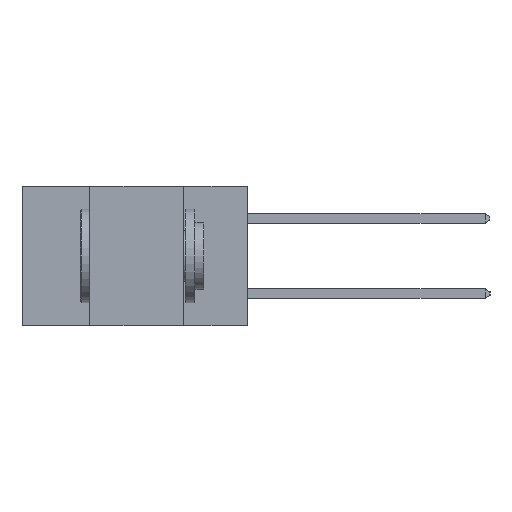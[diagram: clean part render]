
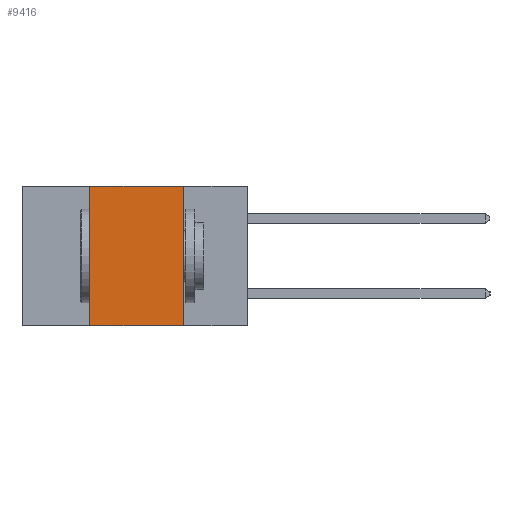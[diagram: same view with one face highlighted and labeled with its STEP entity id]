
A CAD part, left-side view. The second image highlights one B-rep face of the part: STEP entity #9416.
In plain terms, the highlighted planar face has unit normal (-1, 0, 0).
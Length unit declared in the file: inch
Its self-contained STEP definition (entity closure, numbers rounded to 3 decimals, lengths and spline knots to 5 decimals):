
#173 = VERTEX_POINT ( 'NONE', #4301 ) ;
#774 = LINE ( 'NONE', #1029, #2455 ) ;
#1029 = CARTESIAN_POINT ( 'NONE',  ( 0., 0.17, -0.37 ) ) ;
#1184 = CARTESIAN_POINT ( 'NONE',  ( 0., 0.17, 0. ) ) ;
#1533 = PLANE ( 'NONE',  #6991 ) ;
#1644 = LINE ( 'NONE', #10859, #11540 ) ;
#2072 = FACE_OUTER_BOUND ( 'NONE', #11758, .T. ) ;
#2455 = VECTOR ( 'NONE', #7136, 39.37008 ) ;
#2493 = CARTESIAN_POINT ( 'NONE',  ( 0., 0.6, 0. ) ) ;
#2840 = EDGE_CURVE ( 'NONE', #9882, #2846, #774, .T. ) ;
#2846 = VERTEX_POINT ( 'NONE', #10023 ) ;
#2974 = CARTESIAN_POINT ( 'NONE',  ( 0., 0.6, -0.37 ) ) ;
#3141 = LINE ( 'NONE', #6116, #10798 ) ;
#3213 = ORIENTED_EDGE ( 'NONE', *, *, #2840, .F. ) ;
#4301 = CARTESIAN_POINT ( 'NONE',  ( 0., 0.42, -0.37 ) ) ;
#4925 = LINE ( 'NONE', #2974, #12221 ) ;
#5420 = DIRECTION ( 'NONE',  ( 0., 0., -1. ) ) ;
#6071 = EDGE_CURVE ( 'NONE', #173, #8534, #1644, .T. ) ;
#6075 = DIRECTION ( 'NONE',  ( 0., -1., 0. ) ) ;
#6116 = CARTESIAN_POINT ( 'NONE',  ( 0., 0.6, 0. ) ) ;
#6247 = ORIENTED_EDGE ( 'NONE', *, *, #11016, .T. ) ;
#6396 = EDGE_CURVE ( 'NONE', #8534, #9882, #3141, .T. ) ;
#6991 = AXIS2_PLACEMENT_3D ( 'NONE', #2493, #11133, #5420 ) ;
#7136 = DIRECTION ( 'NONE',  ( 0., 0., -1. ) ) ;
#8534 = VERTEX_POINT ( 'NONE', #11732 ) ;
#9416 = ADVANCED_FACE ( 'NONE', ( #2072 ), #1533, .F. ) ;
#9882 = VERTEX_POINT ( 'NONE', #1184 ) ;
#10023 = CARTESIAN_POINT ( 'NONE',  ( 0., 0.17, -0.37 ) ) ;
#10306 = ORIENTED_EDGE ( 'NONE', *, *, #6396, .F. ) ;
#10798 = VECTOR ( 'NONE', #6075, 39.37008 ) ;
#10859 = CARTESIAN_POINT ( 'NONE',  ( 0., 0.42, -0.37 ) ) ;
#10991 = DIRECTION ( 'NONE',  ( 0., 0., 1. ) ) ;
#11016 = EDGE_CURVE ( 'NONE', #173, #2846, #4925, .T. ) ;
#11133 = DIRECTION ( 'NONE',  ( 1., 0., 0. ) ) ;
#11243 = DIRECTION ( 'NONE',  ( 0., -1., 0. ) ) ;
#11540 = VECTOR ( 'NONE', #10991, 39.37008 ) ;
#11732 = CARTESIAN_POINT ( 'NONE',  ( 0., 0.42, 0. ) ) ;
#11758 = EDGE_LOOP ( 'NONE', ( #3213, #10306, #11905, #6247 ) ) ;
#11905 = ORIENTED_EDGE ( 'NONE', *, *, #6071, .F. ) ;
#12221 = VECTOR ( 'NONE', #11243, 39.37008 ) ;
